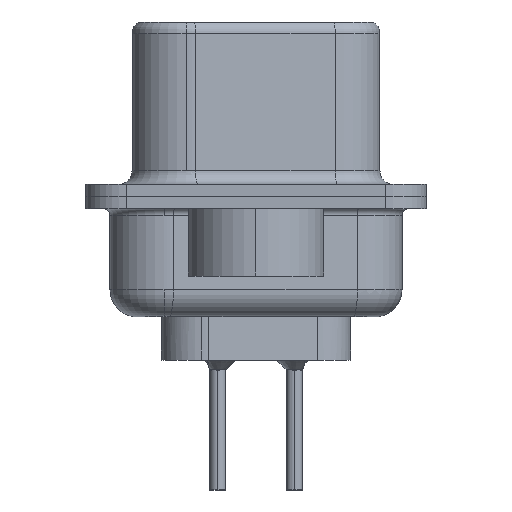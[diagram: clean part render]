
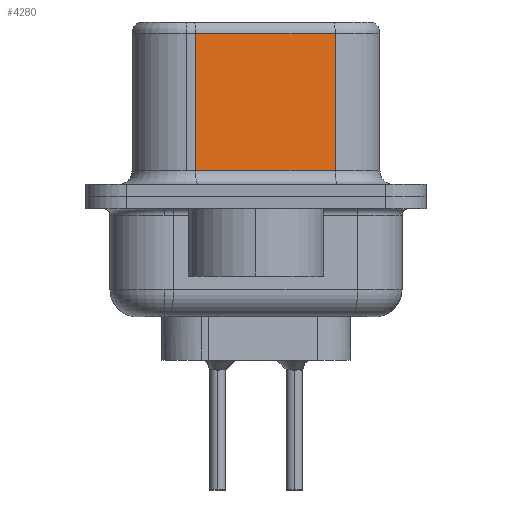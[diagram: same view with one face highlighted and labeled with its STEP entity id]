
A CAD part, left-side view. The second image highlights one B-rep face of the part: STEP entity #4280.
In plain terms, the highlighted planar face has unit normal (-0.985, -0.174, 0).
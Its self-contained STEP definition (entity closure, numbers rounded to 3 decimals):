
#637 = AXIS2_PLACEMENT_3D ( 'NONE', #8446, #12273, #18215 ) ;
#808 = ORIENTED_EDGE ( 'NONE', *, *, #3498, .F. ) ;
#3042 = CARTESIAN_POINT ( 'NONE',  ( 4.58, -2.927, 6.02 ) ) ;
#3051 = EDGE_CURVE ( 'NONE', #16779, #12822, #19719, .T. ) ;
#3498 = EDGE_CURVE ( 'NONE', #13391, #24380, #6699, .T. ) ;
#4280 = ADVANCED_FACE ( 'NONE', ( #8566 ), #24308, .F. ) ;
#4859 = VECTOR ( 'NONE', #11529, 1000. ) ;
#5145 = CARTESIAN_POINT ( 'NONE',  ( 4.58, -2.927, 0.95 ) ) ;
#6573 = DIRECTION ( 'NONE',  ( 0., 0., -1. ) ) ;
#6699 = LINE ( 'NONE', #18636, #17409 ) ;
#7729 = ORIENTED_EDGE ( 'NONE', *, *, #10232, .T. ) ;
#8021 = ORIENTED_EDGE ( 'NONE', *, *, #15236, .T. ) ;
#8171 = DIRECTION ( 'NONE',  ( 0., 0., -1. ) ) ;
#8446 = CARTESIAN_POINT ( 'NONE',  ( 4.58, -2.927, 6.52 ) ) ;
#8566 = FACE_OUTER_BOUND ( 'NONE', #24325, .T. ) ;
#8937 = VECTOR ( 'NONE', #22347, 1000. ) ;
#9009 = LINE ( 'NONE', #3042, #8937 ) ;
#10232 = EDGE_CURVE ( 'NONE', #13391, #16779, #9009, .T. ) ;
#11529 = DIRECTION ( 'NONE',  ( 0.174, -0.985, 0. ) ) ;
#12273 = DIRECTION ( 'NONE',  ( 0.985, 0.174, 0. ) ) ;
#12822 = VERTEX_POINT ( 'NONE', #22361 ) ;
#13391 = VERTEX_POINT ( 'NONE', #24742 ) ;
#15236 = EDGE_CURVE ( 'NONE', #12822, #24380, #22816, .T. ) ;
#16286 = CARTESIAN_POINT ( 'NONE',  ( 4.58, -2.927, 0.95 ) ) ;
#16779 = VERTEX_POINT ( 'NONE', #23232 ) ;
#17409 = VECTOR ( 'NONE', #6573, 1000. ) ;
#17834 = CARTESIAN_POINT ( 'NONE',  ( 3.67, 2.233, 6.52 ) ) ;
#18215 = DIRECTION ( 'NONE',  ( -0.174, 0.985, 0. ) ) ;
#18636 = CARTESIAN_POINT ( 'NONE',  ( 4.58, -2.927, 6.52 ) ) ;
#19719 = LINE ( 'NONE', #17834, #21301 ) ;
#21218 = ORIENTED_EDGE ( 'NONE', *, *, #3051, .T. ) ;
#21301 = VECTOR ( 'NONE', #8171, 1000. ) ;
#22347 = DIRECTION ( 'NONE',  ( -0.174, 0.985, 0. ) ) ;
#22361 = CARTESIAN_POINT ( 'NONE',  ( 3.67, 2.233, 0.95 ) ) ;
#22816 = LINE ( 'NONE', #5145, #4859 ) ;
#23232 = CARTESIAN_POINT ( 'NONE',  ( 3.67, 2.233, 6.02 ) ) ;
#24308 = PLANE ( 'NONE',  #637 ) ;
#24325 = EDGE_LOOP ( 'NONE', ( #808, #7729, #21218, #8021 ) ) ;
#24380 = VERTEX_POINT ( 'NONE', #16286 ) ;
#24742 = CARTESIAN_POINT ( 'NONE',  ( 4.58, -2.927, 6.02 ) ) ;
